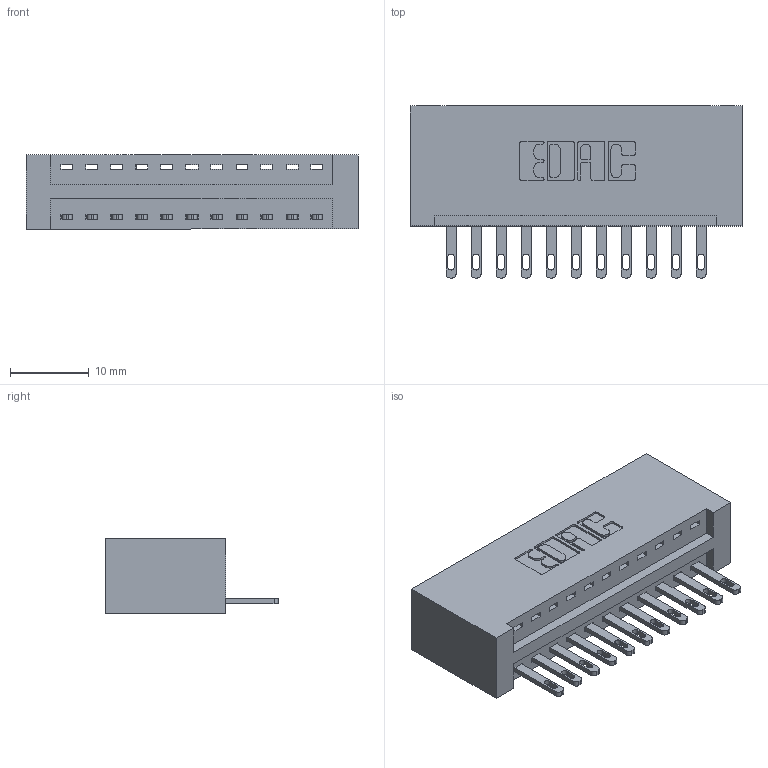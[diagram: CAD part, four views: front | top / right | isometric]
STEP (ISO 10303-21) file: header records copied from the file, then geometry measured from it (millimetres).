
FILE_DESCRIPTION (( 'STEP AP203' ), '1' );
FILE_NAME ('346-011-500-101.STEP', '2022-05-05T00:33:09', ( '' ), ( '' ), 'SwSTEP 2.0', 'SolidWorks 2020', '' );
FILE_SCHEMA (( 'CONFIG_CONTROL_DESIGN' ));
Length unit declared in the file: inch
Products named in the file (3): 346 Part_No Mounting Lugs; 346-011-500-101; 345-292-001_345-293-100
Assembly tree (12 placements, depth 2):
  346-011-500-101
    346 Part_No Mounting Lugs
    345-292-001_345-293-100  x11
Bounding box: 42.16 x 21.84 x 9.4 mm (x, y, z)
Volume: 4378.7 mm3; surface area: 5239 mm2
Topology: 12 solids, 12 shells, 708 faces, 2153 edges, 1434 vertices
Faces by surface type: plane 446, cylinder 262
Entity records: 10653 total; most frequent: CARTESIAN_POINT 1841, ORIENTED_EDGE 1786, DIRECTION 1659, EDGE_CURVE 893, VECTOR 721, LINE 721, VERTEX_POINT 594, AXIS2_PLACEMENT_3D 469
